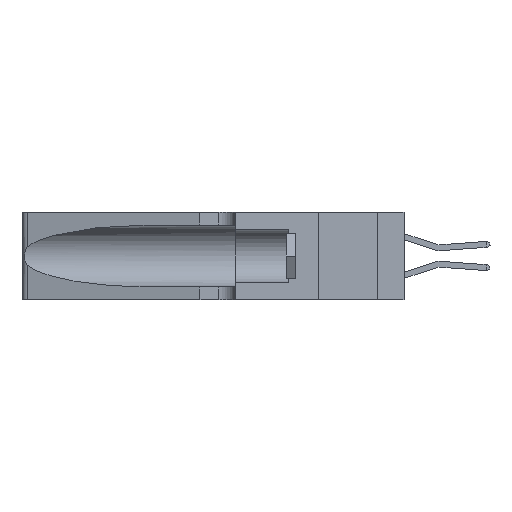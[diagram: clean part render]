
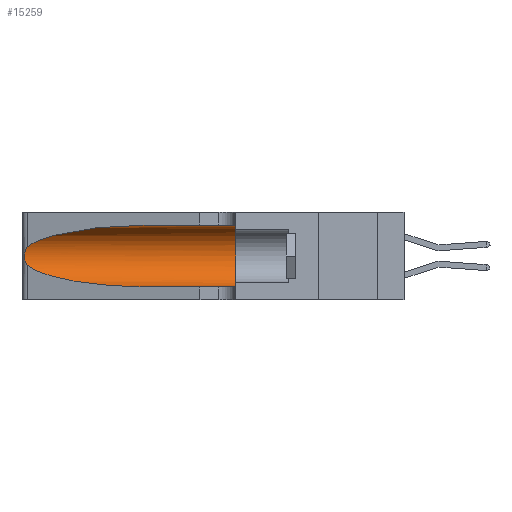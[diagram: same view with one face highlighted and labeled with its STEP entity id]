
A CAD part, left-side view. The second image highlights one B-rep face of the part: STEP entity #15259.
In plain terms, the highlighted cylindrical face has radius 3.308 mm (diameter 6.617 mm), a partial arc.
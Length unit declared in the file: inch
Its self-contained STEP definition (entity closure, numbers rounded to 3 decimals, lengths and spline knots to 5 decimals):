
#335 = CARTESIAN_POINT ( 'NONE',  ( 0.25854, 1.2359, 0.20912 ) ) ;
#1008 = EDGE_LOOP ( 'NONE', ( #8995, #26673, #4702, #25009, #4363, #15248 ) ) ;
#1522 = LINE ( 'NONE', #15386, #19398 ) ;
#1547 = CIRCLE ( 'NONE', #30852, 0.13025 ) ;
#1643 = CARTESIAN_POINT ( 'NONE',  ( 0.1305, 0.72297, 0.31525 ) ) ;
#2383 = AXIS2_PLACEMENT_3D ( 'NONE', #21265, #26136, #28585 ) ;
#2694 = EDGE_CURVE ( 'NONE', #10117, #25444, #22183, .T. ) ;
#2815 = CARTESIAN_POINT ( 'NONE',  ( 0.26075, 1.23896, 0.19203 ) ) ;
#3407 = DIRECTION ( 'NONE',  ( 0., -1., 0. ) ) ;
#3707 = VERTEX_POINT ( 'NONE', #14533 ) ;
#4363 = ORIENTED_EDGE ( 'NONE', *, *, #17094, .F. ) ;
#4702 = ORIENTED_EDGE ( 'NONE', *, *, #2694, .T. ) ;
#4986 = VERTEX_POINT ( 'NONE', #26725 ) ;
#5298 = CARTESIAN_POINT ( 'NONE',  ( 0.26017, 1.23833, 0.17102 ) ) ;
#5777 = DIRECTION ( 'NONE',  ( 0., -1., 0. ) ) ;
#7750 = CARTESIAN_POINT ( 'NONE',  ( 0.25789, 1.23486, 0.15765 ) ) ;
#7926 = CARTESIAN_POINT ( 'NONE',  ( 0.25487, 1.22718, 0.14631 ) ) ;
#8995 = ORIENTED_EDGE ( 'NONE', *, *, #28066, .T. ) ;
#9019 = DIRECTION ( 'NONE',  ( 0., 1., 0. ) ) ;
#10117 = VERTEX_POINT ( 'NONE', #14881 ) ;
#10148 = CARTESIAN_POINT ( 'NONE',  ( 0.25555, 1.22993, 0.14849 ) ) ;
#10336 = CARTESIAN_POINT ( 'NONE',  ( 0.1305, 0.72297, 0.05475 ) ) ;
#12165 = VECTOR ( 'NONE', #3407, 39.37008 ) ;
#12474 = CARTESIAN_POINT ( 'NONE',  ( 0.25555, 1.22994, 0.2215 ) ) ;
#14221 = B_SPLINE_CURVE_WITH_KNOTS ( 'NONE', 3,
 ( #27031, #12474, #29440, #14921, #335, #17383, #2815, #19812, #5298, #22238, #7750, #24681, #10148, #27140 ),
 .UNSPECIFIED., .F., .F.,
 ( 4, 2, 2, 2, 2, 2, 4 ),
 ( 0., 0.00027, 0.00053, 0.00107, 0.0016, 0.00187, 0.00214 ),
 .UNSPECIFIED. ) ;
#14506 = VERTEX_POINT ( 'NONE', #1643 ) ;
#14533 = CARTESIAN_POINT ( 'NONE',  ( 0.1305, 0.35, 0.31525 ) ) ;
#14881 = CARTESIAN_POINT ( 'NONE',  ( 0.25487, 1.22718, 0.14631 ) ) ;
#14921 = CARTESIAN_POINT ( 'NONE',  ( 0.25787, 1.23484, 0.2124 ) ) ;
#15248 = ORIENTED_EDGE ( 'NONE', *, *, #18253, .F. ) ;
#15259 = ADVANCED_FACE ( 'NONE', ( #29707 ), #23289, .F. ) ;
#15386 = CARTESIAN_POINT ( 'NONE',  ( 0.1305, 1.61858, 0.05475 ) ) ;
#16507 = CARTESIAN_POINT ( 'NONE',  ( 0.25487, 1.22718, 0.22369 ) ) ;
#17094 = EDGE_CURVE ( 'NONE', #3707, #22654, #1547, .T. ) ;
#17383 = CARTESIAN_POINT ( 'NONE',  ( 0.26018, 1.23835, 0.19895 ) ) ;
#17570 = CARTESIAN_POINT ( 'NONE',  ( 0.2373, 1.15595, 0.08982 ) ) ;
#18224 = EDGE_CURVE ( 'NONE', #25444, #22654, #1522, .T. ) ;
#18253 = EDGE_CURVE ( 'NONE', #14506, #3707, #25072, .T. ) ;
#19398 = VECTOR ( 'NONE', #5777, 39.37008 ) ;
#19812 = CARTESIAN_POINT ( 'NONE',  ( 0.26075, 1.23896, 0.178 ) ) ;
#20820 = EDGE_CURVE ( 'NONE', #4986, #10117, #14221, .T. ) ;
#21265 = CARTESIAN_POINT ( 'NONE',  ( 0.1305, 1.61858, 0.185 ) ) ;
#22183 =( BOUNDED_CURVE ( )  B_SPLINE_CURVE ( 3, ( #7926, #17570, #24852, #10336 ),
 .UNSPECIFIED., .F., .F. ) 
 B_SPLINE_CURVE_WITH_KNOTS ( ( 4, 4 ),
 ( 3.44316, 4.71239 ),
 .UNSPECIFIED. ) 
 CURVE ( )  GEOMETRIC_REPRESENTATION_ITEM ( )  RATIONAL_B_SPLINE_CURVE ( ( 1., 0.87, 0.87, 1. ) ) 
 REPRESENTATION_ITEM ( '' )  );
#22238 = CARTESIAN_POINT ( 'NONE',  ( 0.25856, 1.23593, 0.16098 ) ) ;
#22654 = VERTEX_POINT ( 'NONE', #24097 ) ;
#23156 =( BOUNDED_CURVE ( )  B_SPLINE_CURVE ( 3, ( #28605, #26158, #31000, #16507 ),
 .UNSPECIFIED., .F., .F. ) 
 B_SPLINE_CURVE_WITH_KNOTS ( ( 4, 4 ),
 ( 1.5708, 2.84003 ),
 .UNSPECIFIED. ) 
 CURVE ( )  GEOMETRIC_REPRESENTATION_ITEM ( )  RATIONAL_B_SPLINE_CURVE ( ( 1., 0.87, 0.87, 1. ) ) 
 REPRESENTATION_ITEM ( '' )  );
#23289 = CYLINDRICAL_SURFACE ( 'NONE', #2383, 0.13025 ) ;
#23525 = CARTESIAN_POINT ( 'NONE',  ( 0.1305, 0.35, 0.185 ) ) ;
#24097 = CARTESIAN_POINT ( 'NONE',  ( 0.1305, 0.35, 0.05475 ) ) ;
#24681 = CARTESIAN_POINT ( 'NONE',  ( 0.25639, 1.23186, 0.15144 ) ) ;
#24852 = CARTESIAN_POINT ( 'NONE',  ( 0.18966, 0.96281, 0.05475 ) ) ;
#25009 = ORIENTED_EDGE ( 'NONE', *, *, #18224, .T. ) ;
#25072 = LINE ( 'NONE', #25158, #12165 ) ;
#25158 = CARTESIAN_POINT ( 'NONE',  ( 0.1305, 1.61858, 0.31525 ) ) ;
#25444 = VERTEX_POINT ( 'NONE', #29527 ) ;
#25967 = DIRECTION ( 'NONE',  ( 0., 0., 1. ) ) ;
#26136 = DIRECTION ( 'NONE',  ( 0., -1., 0. ) ) ;
#26158 = CARTESIAN_POINT ( 'NONE',  ( 0.18966, 0.96281, 0.31525 ) ) ;
#26673 = ORIENTED_EDGE ( 'NONE', *, *, #20820, .T. ) ;
#26725 = CARTESIAN_POINT ( 'NONE',  ( 0.25487, 1.22718, 0.22369 ) ) ;
#27031 = CARTESIAN_POINT ( 'NONE',  ( 0.25487, 1.22718, 0.22369 ) ) ;
#27140 = CARTESIAN_POINT ( 'NONE',  ( 0.25487, 1.22718, 0.14631 ) ) ;
#28066 = EDGE_CURVE ( 'NONE', #14506, #4986, #23156, .T. ) ;
#28585 = DIRECTION ( 'NONE',  ( 0., 0., -1. ) ) ;
#28605 = CARTESIAN_POINT ( 'NONE',  ( 0.1305, 0.72297, 0.31525 ) ) ;
#29440 = CARTESIAN_POINT ( 'NONE',  ( 0.25639, 1.23184, 0.21858 ) ) ;
#29527 = CARTESIAN_POINT ( 'NONE',  ( 0.1305, 0.72297, 0.05475 ) ) ;
#29707 = FACE_OUTER_BOUND ( 'NONE', #1008, .T. ) ;
#30852 = AXIS2_PLACEMENT_3D ( 'NONE', #23525, #9019, #25967 ) ;
#31000 = CARTESIAN_POINT ( 'NONE',  ( 0.2373, 1.15595, 0.28018 ) ) ;
